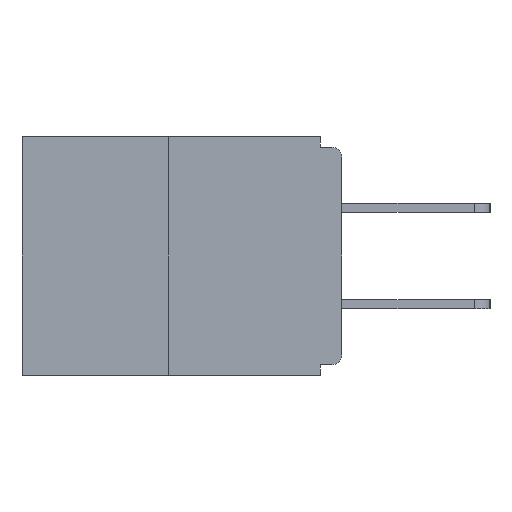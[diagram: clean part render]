
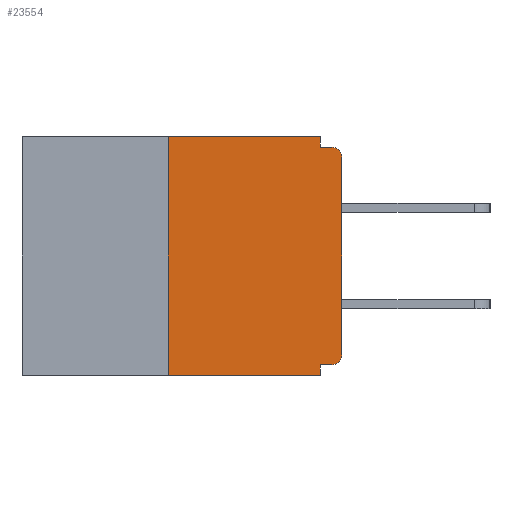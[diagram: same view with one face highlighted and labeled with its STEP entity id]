
A CAD part, left-side view. The second image highlights one B-rep face of the part: STEP entity #23554.
In plain terms, the highlighted planar face has unit normal (-1, 0, 0).
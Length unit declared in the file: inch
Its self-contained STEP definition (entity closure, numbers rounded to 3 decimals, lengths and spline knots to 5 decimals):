
#726 = CARTESIAN_POINT ( 'NONE',  ( 0., 0.015, -0.313 ) ) ;
#1536 = VERTEX_POINT ( 'NONE', #27274 ) ;
#1594 = LINE ( 'NONE', #17944, #13572 ) ;
#1826 = CARTESIAN_POINT ( 'NONE',  ( 0., 0.25, 0. ) ) ;
#1910 = EDGE_CURVE ( 'NONE', #27106, #4199, #22220, .T. ) ;
#2013 = DIRECTION ( 'NONE',  ( 0., 0., 1. ) ) ;
#2479 = CIRCLE ( 'NONE', #7852, 0.015 ) ;
#2882 = AXIS2_PLACEMENT_3D ( 'NONE', #26820, #20787, #25062 ) ;
#3493 = CARTESIAN_POINT ( 'NONE',  ( 0., 0.031, -0.343 ) ) ;
#3674 = ORIENTED_EDGE ( 'NONE', *, *, #10279, .T. ) ;
#4199 = VERTEX_POINT ( 'NONE', #3493 ) ;
#4255 = DIRECTION ( 'NONE',  ( 0., 0., -1. ) ) ;
#4353 = CARTESIAN_POINT ( 'NONE',  ( 0., 0.031, 0. ) ) ;
#4524 = CARTESIAN_POINT ( 'NONE',  ( 0., 0.25, -0.343 ) ) ;
#4723 = DIRECTION ( 'NONE',  ( 0., -1., 0. ) ) ;
#5133 = ORIENTED_EDGE ( 'NONE', *, *, #11066, .F. ) ;
#5393 = FACE_OUTER_BOUND ( 'NONE', #19021, .T. ) ;
#5424 = LINE ( 'NONE', #1826, #18074 ) ;
#6232 = DIRECTION ( 'NONE',  ( 0., 0., 1. ) ) ;
#6966 = VERTEX_POINT ( 'NONE', #8063 ) ;
#7024 = EDGE_CURVE ( 'NONE', #27106, #20829, #5424, .T. ) ;
#7190 = CIRCLE ( 'NONE', #2882, 0.015 ) ;
#7284 = VECTOR ( 'NONE', #6232, 39.37008 ) ;
#7412 = CARTESIAN_POINT ( 'NONE',  ( 0., 0.25, 0. ) ) ;
#7727 = DIRECTION ( 'NONE',  ( 0., 1., 0. ) ) ;
#7852 = AXIS2_PLACEMENT_3D ( 'NONE', #726, #23748, #23842 ) ;
#7932 = ORIENTED_EDGE ( 'NONE', *, *, #10468, .F. ) ;
#8063 = CARTESIAN_POINT ( 'NONE',  ( 0., 0.031, -0.015 ) ) ;
#8306 = ORIENTED_EDGE ( 'NONE', *, *, #10606, .F. ) ;
#8429 = CARTESIAN_POINT ( 'NONE',  ( 0., 0., -0.03 ) ) ;
#8754 = DIRECTION ( 'NONE',  ( 0., -1., 0. ) ) ;
#9332 = VERTEX_POINT ( 'NONE', #8429 ) ;
#9907 = VECTOR ( 'NONE', #24130, 39.37008 ) ;
#10014 = AXIS2_PLACEMENT_3D ( 'NONE', #12469, #12170, #10125 ) ;
#10125 = DIRECTION ( 'NONE',  ( 0., 0., -1. ) ) ;
#10279 = EDGE_CURVE ( 'NONE', #14909, #9332, #15288, .T. ) ;
#10468 = EDGE_CURVE ( 'NONE', #11535, #6966, #24245, .T. ) ;
#10602 = CARTESIAN_POINT ( 'NONE',  ( 0., 0., -0.313 ) ) ;
#10606 = EDGE_CURVE ( 'NONE', #6966, #1536, #17249, .T. ) ;
#11066 = EDGE_CURVE ( 'NONE', #25301, #12894, #20503, .T. ) ;
#11482 = EDGE_CURVE ( 'NONE', #9332, #1536, #7190, .T. ) ;
#11535 = VERTEX_POINT ( 'NONE', #14412 ) ;
#12170 = DIRECTION ( 'NONE',  ( 1., 0., 0. ) ) ;
#12469 = CARTESIAN_POINT ( 'NONE',  ( 0., 0.46, 0. ) ) ;
#12586 = VECTOR ( 'NONE', #7727, 39.37008 ) ;
#12894 = VERTEX_POINT ( 'NONE', #26543 ) ;
#13106 = ORIENTED_EDGE ( 'NONE', *, *, #22369, .T. ) ;
#13572 = VECTOR ( 'NONE', #26114, 39.37008 ) ;
#13941 = VECTOR ( 'NONE', #4723, 39.37008 ) ;
#14066 = CARTESIAN_POINT ( 'NONE',  ( 0., 0., -0.328 ) ) ;
#14095 = ORIENTED_EDGE ( 'NONE', *, *, #7024, .F. ) ;
#14412 = CARTESIAN_POINT ( 'NONE',  ( 0., 0.031, 0. ) ) ;
#14551 = CARTESIAN_POINT ( 'NONE',  ( 0., 0.46, 0. ) ) ;
#14909 = VERTEX_POINT ( 'NONE', #10602 ) ;
#15220 = CARTESIAN_POINT ( 'NONE',  ( 0., 0.015, -0.328 ) ) ;
#15244 = CARTESIAN_POINT ( 'NONE',  ( 0., 0.46, -0.343 ) ) ;
#15261 = ORIENTED_EDGE ( 'NONE', *, *, #18031, .F. ) ;
#15288 = LINE ( 'NONE', #21088, #7284 ) ;
#15696 = ORIENTED_EDGE ( 'NONE', *, *, #11482, .T. ) ;
#16814 = ORIENTED_EDGE ( 'NONE', *, *, #20195, .F. ) ;
#17249 = LINE ( 'NONE', #22077, #9907 ) ;
#17944 = CARTESIAN_POINT ( 'NONE',  ( 0., 0.031, -0.343 ) ) ;
#18031 = EDGE_CURVE ( 'NONE', #20829, #11535, #18627, .T. ) ;
#18071 = ORIENTED_EDGE ( 'NONE', *, *, #1910, .T. ) ;
#18074 = VECTOR ( 'NONE', #2013, 39.37008 ) ;
#18581 = VECTOR ( 'NONE', #4255, 39.37008 ) ;
#18627 = LINE ( 'NONE', #14551, #23671 ) ;
#19021 = EDGE_LOOP ( 'NONE', ( #15261, #14095, #18071, #16814, #5133, #13106, #3674, #15696, #8306, #7932 ) ) ;
#20195 = EDGE_CURVE ( 'NONE', #12894, #4199, #1594, .T. ) ;
#20503 = LINE ( 'NONE', #14066, #12586 ) ;
#20787 = DIRECTION ( 'NONE',  ( -1., 0., 0. ) ) ;
#20829 = VERTEX_POINT ( 'NONE', #7412 ) ;
#21088 = CARTESIAN_POINT ( 'NONE',  ( 0., 0., 0. ) ) ;
#22077 = CARTESIAN_POINT ( 'NONE',  ( 0., 0., -0.015 ) ) ;
#22220 = LINE ( 'NONE', #15244, #13941 ) ;
#22369 = EDGE_CURVE ( 'NONE', #25301, #14909, #2479, .T. ) ;
#22961 = PLANE ( 'NONE',  #10014 ) ;
#23554 = ADVANCED_FACE ( 'NONE', ( #5393 ), #22961, .F. ) ;
#23671 = VECTOR ( 'NONE', #8754, 39.37008 ) ;
#23748 = DIRECTION ( 'NONE',  ( -1., 0., 0. ) ) ;
#23842 = DIRECTION ( 'NONE',  ( 0., 0., -1. ) ) ;
#24130 = DIRECTION ( 'NONE',  ( 0., -1., 0. ) ) ;
#24245 = LINE ( 'NONE', #4353, #18581 ) ;
#25062 = DIRECTION ( 'NONE',  ( 0., 0., -1. ) ) ;
#25301 = VERTEX_POINT ( 'NONE', #15220 ) ;
#26114 = DIRECTION ( 'NONE',  ( 0., 0., -1. ) ) ;
#26543 = CARTESIAN_POINT ( 'NONE',  ( 0., 0.031, -0.328 ) ) ;
#26820 = CARTESIAN_POINT ( 'NONE',  ( 0., 0.015, -0.03 ) ) ;
#27106 = VERTEX_POINT ( 'NONE', #4524 ) ;
#27274 = CARTESIAN_POINT ( 'NONE',  ( 0., 0.015, -0.015 ) ) ;
